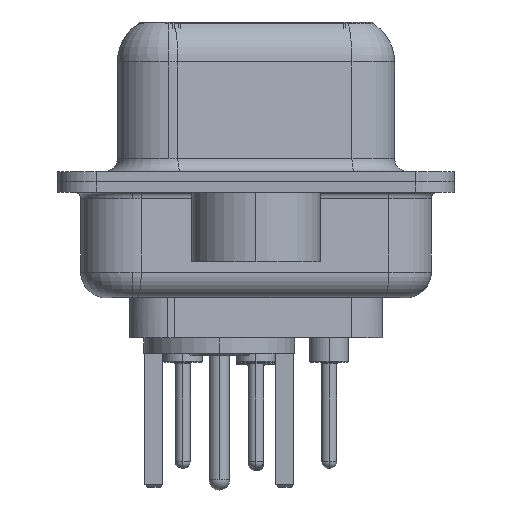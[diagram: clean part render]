
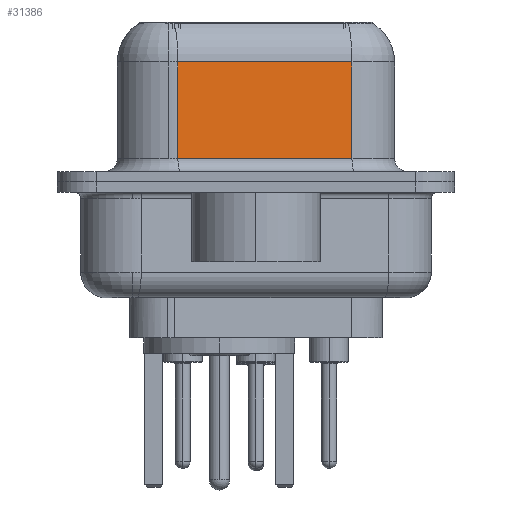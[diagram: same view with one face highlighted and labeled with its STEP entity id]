
A CAD part, left-side view. The second image highlights one B-rep face of the part: STEP entity #31386.
In plain terms, the highlighted planar face has unit normal (-0.985, -0.174, 0).
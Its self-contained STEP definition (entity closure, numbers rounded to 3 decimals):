
#1391 = LINE ( 'NONE', #8235, #23931 ) ;
#1900 = CARTESIAN_POINT ( 'NONE',  ( 5.621, -3.722, 4.65 ) ) ;
#4227 = LINE ( 'NONE', #18411, #23924 ) ;
#5436 = FACE_OUTER_BOUND ( 'NONE', #18074, .T. ) ;
#6772 = ORIENTED_EDGE ( 'NONE', *, *, #10430, .T. ) ;
#7222 = ORIENTED_EDGE ( 'NONE', *, *, #18741, .F. ) ;
#8235 = CARTESIAN_POINT ( 'NONE',  ( 4.43, 3.028, 6.4 ) ) ;
#8359 = VECTOR ( 'NONE', #30432, 1000. ) ;
#9039 = CARTESIAN_POINT ( 'NONE',  ( 4.43, 3.028, 4.65 ) ) ;
#9462 = CARTESIAN_POINT ( 'NONE',  ( 5.621, -3.722, 0.9 ) ) ;
#9784 = VERTEX_POINT ( 'NONE', #9462 ) ;
#9848 = ORIENTED_EDGE ( 'NONE', *, *, #24822, .T. ) ;
#10430 = EDGE_CURVE ( 'NONE', #21741, #14818, #24777, .T. ) ;
#10519 = DIRECTION ( 'NONE',  ( 0.174, -0.985, 0. ) ) ;
#11532 = PLANE ( 'NONE',  #25358 ) ;
#12956 = DIRECTION ( 'NONE',  ( 0., 0., -1. ) ) ;
#14818 = VERTEX_POINT ( 'NONE', #9039 ) ;
#18074 = EDGE_LOOP ( 'NONE', ( #7222, #6772, #9848, #23751 ) ) ;
#18411 = CARTESIAN_POINT ( 'NONE',  ( 5.621, -3.722, 0.9 ) ) ;
#18741 = EDGE_CURVE ( 'NONE', #21741, #9784, #28808, .T. ) ;
#20091 = CARTESIAN_POINT ( 'NONE',  ( 5.621, -3.722, 6.4 ) ) ;
#21741 = VERTEX_POINT ( 'NONE', #30746 ) ;
#21776 = CARTESIAN_POINT ( 'NONE',  ( 4.43, 3.028, 0.9 ) ) ;
#21797 = VECTOR ( 'NONE', #24915, 1000. ) ;
#22524 = DIRECTION ( 'NONE',  ( 0.985, 0.174, 0. ) ) ;
#23751 = ORIENTED_EDGE ( 'NONE', *, *, #31033, .T. ) ;
#23924 = VECTOR ( 'NONE', #10519, 1000. ) ;
#23931 = VECTOR ( 'NONE', #12956, 1000. ) ;
#24777 = LINE ( 'NONE', #1900, #8359 ) ;
#24822 = EDGE_CURVE ( 'NONE', #14818, #30405, #1391, .T. ) ;
#24915 = DIRECTION ( 'NONE',  ( 0., 0., -1. ) ) ;
#25358 = AXIS2_PLACEMENT_3D ( 'NONE', #27379, #22524, #29896 ) ;
#27379 = CARTESIAN_POINT ( 'NONE',  ( 5.621, -3.722, 6.4 ) ) ;
#28808 = LINE ( 'NONE', #20091, #21797 ) ;
#29896 = DIRECTION ( 'NONE',  ( -0.174, 0.985, 0. ) ) ;
#30405 = VERTEX_POINT ( 'NONE', #21776 ) ;
#30432 = DIRECTION ( 'NONE',  ( -0.174, 0.985, 0. ) ) ;
#30746 = CARTESIAN_POINT ( 'NONE',  ( 5.621, -3.722, 4.65 ) ) ;
#31033 = EDGE_CURVE ( 'NONE', #30405, #9784, #4227, .T. ) ;
#31386 = ADVANCED_FACE ( 'NONE', ( #5436 ), #11532, .F. ) ;
